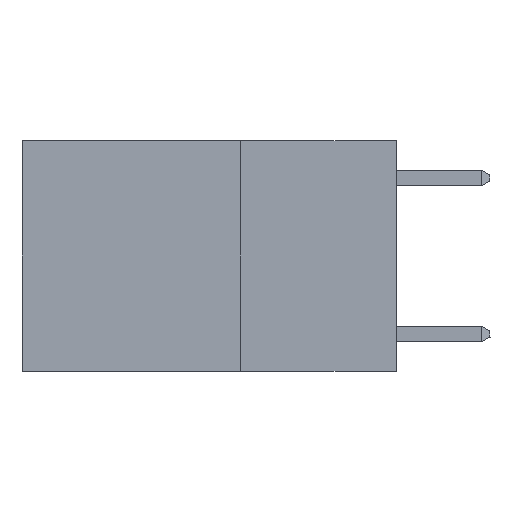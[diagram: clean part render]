
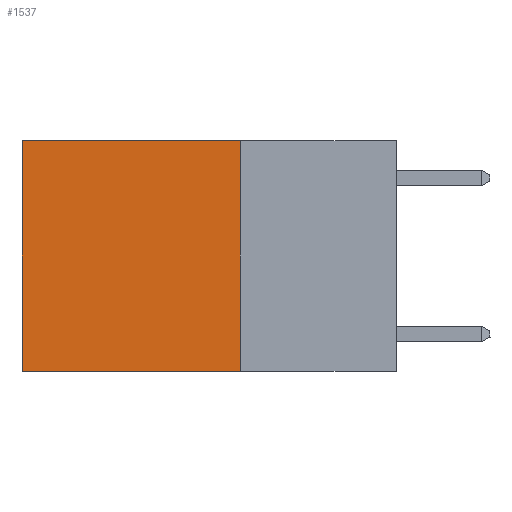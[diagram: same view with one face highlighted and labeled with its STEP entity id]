
A CAD part, left-side view. The second image highlights one B-rep face of the part: STEP entity #1537.
In plain terms, the highlighted planar face has unit normal (-1, 0, 0).
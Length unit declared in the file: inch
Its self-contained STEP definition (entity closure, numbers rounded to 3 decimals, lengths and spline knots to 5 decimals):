
#391 = AXIS2_PLACEMENT_3D ( 'NONE', #7427, #8357, #5692 ) ;
#493 = VECTOR ( 'NONE', #3807, 39.37008 ) ;
#1073 = VERTEX_POINT ( 'NONE', #8456 ) ;
#1537 = ADVANCED_FACE ( 'NONE', ( #9774 ), #3828, .F. ) ;
#2620 = EDGE_LOOP ( 'NONE', ( #3076, #7884, #3342, #8181 ) ) ;
#2979 = LINE ( 'NONE', #5873, #9810 ) ;
#3076 = ORIENTED_EDGE ( 'NONE', *, *, #5092, .T. ) ;
#3119 = LINE ( 'NONE', #4716, #493 ) ;
#3342 = ORIENTED_EDGE ( 'NONE', *, *, #10825, .F. ) ;
#3510 = EDGE_CURVE ( 'NONE', #5032, #8244, #11364, .T. ) ;
#3807 = DIRECTION ( 'NONE',  ( 0., 0., -1. ) ) ;
#3828 = PLANE ( 'NONE',  #391 ) ;
#4716 = CARTESIAN_POINT ( 'NONE',  ( 0.2625, 0.6, 0. ) ) ;
#4764 = VERTEX_POINT ( 'NONE', #8818 ) ;
#5032 = VERTEX_POINT ( 'NONE', #11519 ) ;
#5092 = EDGE_CURVE ( 'NONE', #8244, #4764, #3119, .T. ) ;
#5473 = VECTOR ( 'NONE', #11359, 39.37008 ) ;
#5692 = DIRECTION ( 'NONE',  ( 0., 0., -1. ) ) ;
#5873 = CARTESIAN_POINT ( 'NONE',  ( 0.2625, 0.25, 0. ) ) ;
#6849 = VECTOR ( 'NONE', #10923, 39.37008 ) ;
#7427 = CARTESIAN_POINT ( 'NONE',  ( 0.2625, 0.25, 0. ) ) ;
#7884 = ORIENTED_EDGE ( 'NONE', *, *, #8184, .F. ) ;
#8071 = CARTESIAN_POINT ( 'NONE',  ( 0.2625, 0.25, -0.37 ) ) ;
#8117 = CARTESIAN_POINT ( 'NONE',  ( 0.2625, 0.6, 0. ) ) ;
#8181 = ORIENTED_EDGE ( 'NONE', *, *, #3510, .T. ) ;
#8184 = EDGE_CURVE ( 'NONE', #1073, #4764, #8692, .T. ) ;
#8244 = VERTEX_POINT ( 'NONE', #8117 ) ;
#8357 = DIRECTION ( 'NONE',  ( 1., 0., 0. ) ) ;
#8456 = CARTESIAN_POINT ( 'NONE',  ( 0.2625, 0.25, -0.37 ) ) ;
#8584 = DIRECTION ( 'NONE',  ( 0., 0., -1. ) ) ;
#8692 = LINE ( 'NONE', #8071, #5473 ) ;
#8818 = CARTESIAN_POINT ( 'NONE',  ( 0.2625, 0.6, -0.37 ) ) ;
#9305 = CARTESIAN_POINT ( 'NONE',  ( 0.2625, 0.25, 0. ) ) ;
#9774 = FACE_OUTER_BOUND ( 'NONE', #2620, .T. ) ;
#9810 = VECTOR ( 'NONE', #8584, 39.37008 ) ;
#10825 = EDGE_CURVE ( 'NONE', #5032, #1073, #2979, .T. ) ;
#10923 = DIRECTION ( 'NONE',  ( 0., 1., 0. ) ) ;
#11359 = DIRECTION ( 'NONE',  ( 0., 1., 0. ) ) ;
#11364 = LINE ( 'NONE', #9305, #6849 ) ;
#11519 = CARTESIAN_POINT ( 'NONE',  ( 0.2625, 0.25, 0. ) ) ;
